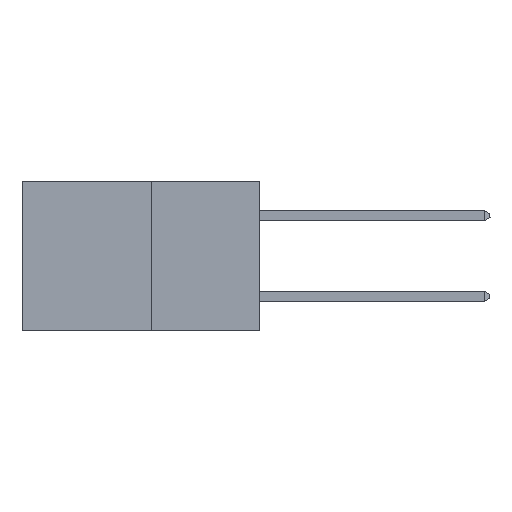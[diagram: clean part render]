
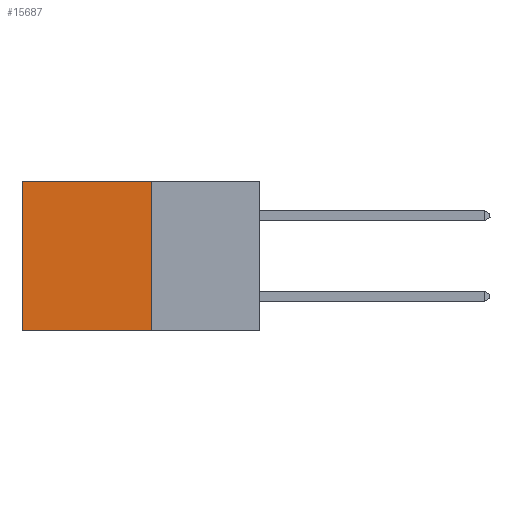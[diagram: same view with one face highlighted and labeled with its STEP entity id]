
A CAD part, left-side view. The second image highlights one B-rep face of the part: STEP entity #15687.
In plain terms, the highlighted planar face has unit normal (-1, 0, 0).
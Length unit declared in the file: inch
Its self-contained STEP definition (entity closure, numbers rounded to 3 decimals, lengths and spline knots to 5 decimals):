
#680 = LINE ( 'NONE', #3766, #12325 ) ;
#1345 = EDGE_LOOP ( 'NONE', ( #9010, #7508, #13959, #14739 ) ) ;
#1772 = DIRECTION ( 'NONE',  ( 0., 1., 0. ) ) ;
#1776 = EDGE_CURVE ( 'NONE', #15009, #13295, #19660, .T. ) ;
#1795 = CARTESIAN_POINT ( 'NONE',  ( 0.277, 0.27, 0. ) ) ;
#1908 = EDGE_CURVE ( 'NONE', #13295, #3051, #14920, .T. ) ;
#2439 = AXIS2_PLACEMENT_3D ( 'NONE', #6119, #18323, #9348 ) ;
#3051 = VERTEX_POINT ( 'NONE', #15895 ) ;
#3620 = DIRECTION ( 'NONE',  ( 0., 1., 0. ) ) ;
#3766 = CARTESIAN_POINT ( 'NONE',  ( 0.277, 0.27, -0.37 ) ) ;
#5179 = VECTOR ( 'NONE', #8092, 39.37008 ) ;
#6119 = CARTESIAN_POINT ( 'NONE',  ( 0.277, 0.27, -0.37 ) ) ;
#7190 = FACE_OUTER_BOUND ( 'NONE', #1345, .T. ) ;
#7508 = ORIENTED_EDGE ( 'NONE', *, *, #16043, .F. ) ;
#7696 = CARTESIAN_POINT ( 'NONE',  ( 0.277, 0.27, -0.37 ) ) ;
#8092 = DIRECTION ( 'NONE',  ( 0., 0., -1. ) ) ;
#8143 = CARTESIAN_POINT ( 'NONE',  ( 0.277, 0.59, -0.37 ) ) ;
#8445 = CARTESIAN_POINT ( 'NONE',  ( 0.277, 0.27, -0.37 ) ) ;
#8767 = EDGE_CURVE ( 'NONE', #15009, #15255, #15371, .T. ) ;
#9010 = ORIENTED_EDGE ( 'NONE', *, *, #1908, .T. ) ;
#9348 = DIRECTION ( 'NONE',  ( 0., 0., -1. ) ) ;
#10850 = DIRECTION ( 'NONE',  ( 0., 0., -1. ) ) ;
#12325 = VECTOR ( 'NONE', #3620, 39.37008 ) ;
#13295 = VERTEX_POINT ( 'NONE', #18120 ) ;
#13959 = ORIENTED_EDGE ( 'NONE', *, *, #8767, .F. ) ;
#14739 = ORIENTED_EDGE ( 'NONE', *, *, #1776, .T. ) ;
#14920 = LINE ( 'NONE', #8143, #5179 ) ;
#15009 = VERTEX_POINT ( 'NONE', #19568 ) ;
#15255 = VERTEX_POINT ( 'NONE', #8445 ) ;
#15371 = LINE ( 'NONE', #7696, #19637 ) ;
#15687 = ADVANCED_FACE ( 'NONE', ( #7190 ), #16878, .F. ) ;
#15895 = CARTESIAN_POINT ( 'NONE',  ( 0.277, 0.59, -0.37 ) ) ;
#16043 = EDGE_CURVE ( 'NONE', #15255, #3051, #680, .T. ) ;
#16317 = VECTOR ( 'NONE', #1772, 39.37008 ) ;
#16878 = PLANE ( 'NONE',  #2439 ) ;
#18120 = CARTESIAN_POINT ( 'NONE',  ( 0.277, 0.59, 0. ) ) ;
#18323 = DIRECTION ( 'NONE',  ( 1., 0., 0. ) ) ;
#19568 = CARTESIAN_POINT ( 'NONE',  ( 0.277, 0.27, 0. ) ) ;
#19637 = VECTOR ( 'NONE', #10850, 39.37008 ) ;
#19660 = LINE ( 'NONE', #1795, #16317 ) ;
